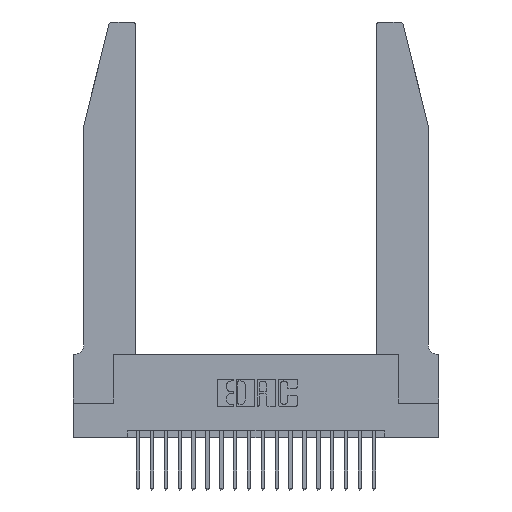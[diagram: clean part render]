
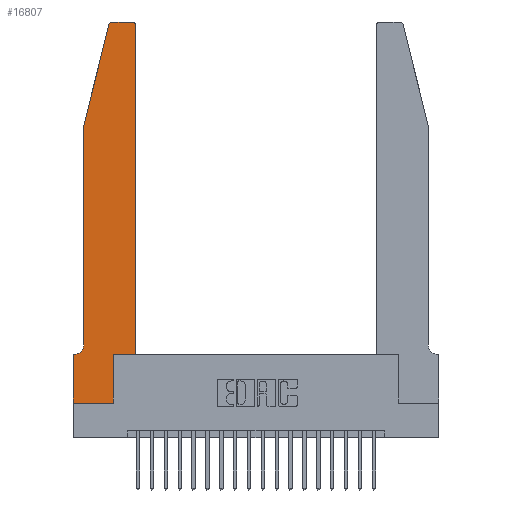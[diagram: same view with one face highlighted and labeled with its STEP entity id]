
A CAD part, top view. The second image highlights one B-rep face of the part: STEP entity #16807.
In plain terms, the highlighted planar face has unit normal (0, 0, 1).
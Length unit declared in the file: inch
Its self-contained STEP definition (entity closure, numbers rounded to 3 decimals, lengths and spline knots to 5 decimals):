
#126 = CIRCLE ( 'NONE', #20326, 0.03 ) ;
#146 = AXIS2_PLACEMENT_3D ( 'NONE', #7652, #21310, #11078 ) ;
#503 = CARTESIAN_POINT ( 'NONE',  ( 0., 0., 0.37 ) ) ;
#520 = ORIENTED_EDGE ( 'NONE', *, *, #14454, .T. ) ;
#706 = EDGE_CURVE ( 'NONE', #4372, #9716, #5827, .T. ) ;
#920 = DIRECTION ( 'NONE',  ( 0., 0., 1. ) ) ;
#1063 = ORIENTED_EDGE ( 'NONE', *, *, #19183, .T. ) ;
#1248 = VECTOR ( 'NONE', #7146, 39.37008 ) ;
#1573 = EDGE_CURVE ( 'NONE', #20811, #12641, #3388, .T. ) ;
#1676 = CARTESIAN_POINT ( 'NONE',  ( 0.0755, 0.35, 0.37 ) ) ;
#1810 = LINE ( 'NONE', #20268, #14918 ) ;
#2251 = DIRECTION ( 'NONE',  ( 1., 0., 0. ) ) ;
#2589 = LINE ( 'NONE', #503, #20203 ) ;
#2851 = CARTESIAN_POINT ( 'NONE',  ( 0.2865, 0.35, 0.37 ) ) ;
#3053 = EDGE_CURVE ( 'NONE', #9716, #9972, #12381, .T. ) ;
#3063 = DIRECTION ( 'NONE',  ( 1., 0., 0. ) ) ;
#3184 = DIRECTION ( 'NONE',  ( -0.239, -0.971, 0. ) ) ;
#3388 = CIRCLE ( 'NONE', #21494, 0.07 ) ;
#3591 = LINE ( 'NONE', #1676, #21186 ) ;
#3961 = LINE ( 'NONE', #5514, #21008 ) ;
#4011 = LINE ( 'NONE', #8234, #21598 ) ;
#4124 = AXIS2_PLACEMENT_3D ( 'NONE', #11177, #920, #12901 ) ;
#4372 = VERTEX_POINT ( 'NONE', #19050 ) ;
#4389 = CARTESIAN_POINT ( 'NONE',  ( 0., 0., 0.37 ) ) ;
#5514 = CARTESIAN_POINT ( 'NONE',  ( 0.2605, 2.75, 0.37 ) ) ;
#5653 = CARTESIAN_POINT ( 'NONE',  ( 0., 0.35, 0.37 ) ) ;
#5663 = ORIENTED_EDGE ( 'NONE', *, *, #18735, .T. ) ;
#5827 = LINE ( 'NONE', #7140, #1248 ) ;
#5876 = DIRECTION ( 'NONE',  ( 0., 0., 1. ) ) ;
#6449 = VERTEX_POINT ( 'NONE', #21412 ) ;
#6561 = VERTEX_POINT ( 'NONE', #13135 ) ;
#7140 = CARTESIAN_POINT ( 'NONE',  ( 0.2865, 0.35, 0.37 ) ) ;
#7146 = DIRECTION ( 'NONE',  ( 0., 1., 0. ) ) ;
#7232 = ORIENTED_EDGE ( 'NONE', *, *, #11478, .T. ) ;
#7273 = CARTESIAN_POINT ( 'NONE',  ( 0.0055, 0.35, 0.37 ) ) ;
#7652 = CARTESIAN_POINT ( 'NONE',  ( 0., 0.35, 0.37 ) ) ;
#7847 = VECTOR ( 'NONE', #3063, 39.37008 ) ;
#8234 = CARTESIAN_POINT ( 'NONE',  ( 0.0755, 2., 0.37 ) ) ;
#8469 = VERTEX_POINT ( 'NONE', #5653 ) ;
#9716 = VERTEX_POINT ( 'NONE', #2851 ) ;
#9972 = VERTEX_POINT ( 'NONE', #18950 ) ;
#10235 = VECTOR ( 'NONE', #18497, 39.37008 ) ;
#10318 = EDGE_CURVE ( 'NONE', #8469, #11650, #1810, .T. ) ;
#10701 = ORIENTED_EDGE ( 'NONE', *, *, #1573, .T. ) ;
#10750 = FACE_OUTER_BOUND ( 'NONE', #13613, .T. ) ;
#11078 = DIRECTION ( 'NONE',  ( 1., 0., 0. ) ) ;
#11177 = CARTESIAN_POINT ( 'NONE',  ( 0.284, 2.72, 0.37 ) ) ;
#11315 = LINE ( 'NONE', #15061, #10235 ) ;
#11478 = EDGE_CURVE ( 'NONE', #11650, #4372, #2589, .T. ) ;
#11551 = CARTESIAN_POINT ( 'NONE',  ( 0.4505, 0.35, 0.37 ) ) ;
#11650 = VERTEX_POINT ( 'NONE', #4389 ) ;
#11759 = CARTESIAN_POINT ( 'NONE',  ( 0.4505, 2.72, 0.37 ) ) ;
#11777 = ORIENTED_EDGE ( 'NONE', *, *, #706, .T. ) ;
#12199 = DIRECTION ( 'NONE',  ( -1., 0., 0. ) ) ;
#12216 = DIRECTION ( 'NONE',  ( 0., 0., -1. ) ) ;
#12268 = DIRECTION ( 'NONE',  ( -1., 0., 0. ) ) ;
#12313 = ORIENTED_EDGE ( 'NONE', *, *, #3053, .T. ) ;
#12381 = LINE ( 'NONE', #11551, #7847 ) ;
#12641 = VERTEX_POINT ( 'NONE', #7273 ) ;
#12782 = CARTESIAN_POINT ( 'NONE',  ( 0.0055, 0.42, 0.37 ) ) ;
#12901 = DIRECTION ( 'NONE',  ( 1., 0., 0. ) ) ;
#13135 = CARTESIAN_POINT ( 'NONE',  ( 0.4205, 2.75, 0.37 ) ) ;
#13280 = DIRECTION ( 'NONE',  ( 0., 1., 0. ) ) ;
#13490 = DIRECTION ( 'NONE',  ( 0., -1., 0. ) ) ;
#13613 = EDGE_LOOP ( 'NONE', ( #520, #1063, #5663, #19254, #10701, #15245, #20317, #7232, #11777, #12313, #21391, #17940 ) ) ;
#13809 = CARTESIAN_POINT ( 'NONE',  ( 0.0755, 0.42, 0.37 ) ) ;
#14454 = EDGE_CURVE ( 'NONE', #6561, #20492, #3961, .T. ) ;
#14623 = EDGE_CURVE ( 'NONE', #19410, #6561, #126, .T. ) ;
#14649 = CIRCLE ( 'NONE', #4124, 0.03 ) ;
#14918 = VECTOR ( 'NONE', #13490, 39.37008 ) ;
#15061 = CARTESIAN_POINT ( 'NONE',  ( 0.0755, 2., 0.37 ) ) ;
#15245 = ORIENTED_EDGE ( 'NONE', *, *, #16493, .T. ) ;
#15317 = LINE ( 'NONE', #21846, #19857 ) ;
#15347 = DIRECTION ( 'NONE',  ( -1., 0., 0. ) ) ;
#16084 = CARTESIAN_POINT ( 'NONE',  ( 0.4205, 2.72, 0.37 ) ) ;
#16169 = PLANE ( 'NONE',  #146 ) ;
#16353 = EDGE_CURVE ( 'NONE', #9972, #19410, #15317, .T. ) ;
#16361 = EDGE_CURVE ( 'NONE', #6449, #20811, #11315, .T. ) ;
#16493 = EDGE_CURVE ( 'NONE', #12641, #8469, #3591, .T. ) ;
#16759 = CARTESIAN_POINT ( 'NONE',  ( 0.25487, 2.72718, 0.37 ) ) ;
#16807 = ADVANCED_FACE ( 'NONE', ( #10750 ), #16169, .T. ) ;
#17018 = VERTEX_POINT ( 'NONE', #16759 ) ;
#17798 = DIRECTION ( 'NONE',  ( 1., 0., 0. ) ) ;
#17940 = ORIENTED_EDGE ( 'NONE', *, *, #14623, .T. ) ;
#18497 = DIRECTION ( 'NONE',  ( 0., -1., 0. ) ) ;
#18735 = EDGE_CURVE ( 'NONE', #17018, #6449, #4011, .T. ) ;
#18950 = CARTESIAN_POINT ( 'NONE',  ( 0.4505, 0.35, 0.37 ) ) ;
#19050 = CARTESIAN_POINT ( 'NONE',  ( 0.2865, 0., 0.37 ) ) ;
#19183 = EDGE_CURVE ( 'NONE', #20492, #17018, #14649, .T. ) ;
#19254 = ORIENTED_EDGE ( 'NONE', *, *, #16361, .T. ) ;
#19410 = VERTEX_POINT ( 'NONE', #11759 ) ;
#19857 = VECTOR ( 'NONE', #13280, 39.37008 ) ;
#20203 = VECTOR ( 'NONE', #2251, 39.37008 ) ;
#20268 = CARTESIAN_POINT ( 'NONE',  ( 0., 0., 0.37 ) ) ;
#20317 = ORIENTED_EDGE ( 'NONE', *, *, #10318, .T. ) ;
#20326 = AXIS2_PLACEMENT_3D ( 'NONE', #16084, #5876, #17798 ) ;
#20492 = VERTEX_POINT ( 'NONE', #21418 ) ;
#20811 = VERTEX_POINT ( 'NONE', #13809 ) ;
#21008 = VECTOR ( 'NONE', #12268, 39.37008 ) ;
#21186 = VECTOR ( 'NONE', #15347, 39.37008 ) ;
#21310 = DIRECTION ( 'NONE',  ( 0., 0., 1. ) ) ;
#21391 = ORIENTED_EDGE ( 'NONE', *, *, #16353, .T. ) ;
#21412 = CARTESIAN_POINT ( 'NONE',  ( 0.0755, 2., 0.37 ) ) ;
#21418 = CARTESIAN_POINT ( 'NONE',  ( 0.284, 2.75, 0.37 ) ) ;
#21494 = AXIS2_PLACEMENT_3D ( 'NONE', #12782, #12216, #12199 ) ;
#21598 = VECTOR ( 'NONE', #3184, 39.37008 ) ;
#21846 = CARTESIAN_POINT ( 'NONE',  ( 0.4505, 0.35, 0.37 ) ) ;
